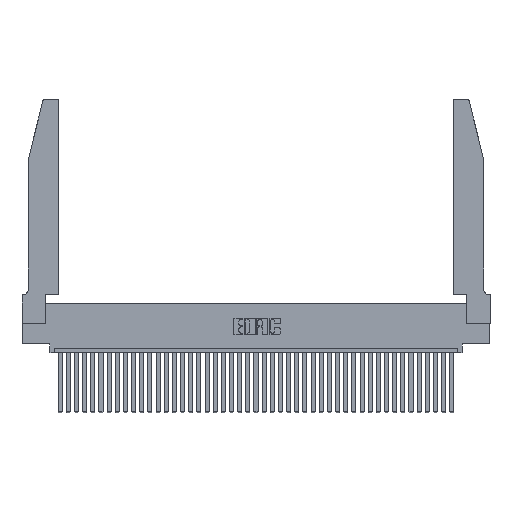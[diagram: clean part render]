
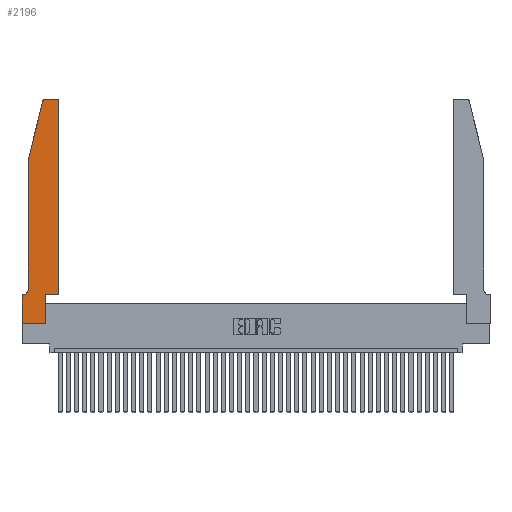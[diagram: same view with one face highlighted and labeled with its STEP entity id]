
A CAD part, top view. The second image highlights one B-rep face of the part: STEP entity #2196.
In plain terms, the highlighted planar face has unit normal (0, 0, 1).
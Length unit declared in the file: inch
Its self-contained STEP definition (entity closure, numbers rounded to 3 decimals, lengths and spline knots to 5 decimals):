
#500 = LINE ( 'NONE', #21204, #25167 ) ;
#563 = VERTEX_POINT ( 'NONE', #28806 ) ;
#975 = VECTOR ( 'NONE', #16520, 39.37008 ) ;
#1058 = EDGE_CURVE ( 'NONE', #33001, #15711, #18841, .T. ) ;
#1195 = ORIENTED_EDGE ( 'NONE', *, *, #20455, .T. ) ;
#1281 = EDGE_CURVE ( 'NONE', #563, #17294, #22710, .T. ) ;
#1528 = LINE ( 'NONE', #12996, #8435 ) ;
#2046 = ORIENTED_EDGE ( 'NONE', *, *, #39128, .T. ) ;
#2063 = CARTESIAN_POINT ( 'NONE',  ( 0.0755, 2., 0.37 ) ) ;
#2196 = ADVANCED_FACE ( 'NONE', ( #28555 ), #40489, .T. ) ;
#2417 = DIRECTION ( 'NONE',  ( 0., -1., 0. ) ) ;
#2602 = DIRECTION ( 'NONE',  ( 1., 0., 0. ) ) ;
#2818 = EDGE_CURVE ( 'NONE', #26857, #16723, #28489, .T. ) ;
#2832 = VERTEX_POINT ( 'NONE', #28249 ) ;
#2904 = ORIENTED_EDGE ( 'NONE', *, *, #22901, .T. ) ;
#3601 = CARTESIAN_POINT ( 'NONE',  ( 0.4505, 2.72, 0.37 ) ) ;
#4555 = EDGE_LOOP ( 'NONE', ( #2046, #27588, #8242, #13782, #1195, #13633, #35227, #15283, #33501, #24519, #2904, #5033 ) ) ;
#5033 = ORIENTED_EDGE ( 'NONE', *, *, #39528, .T. ) ;
#5931 = CIRCLE ( 'NONE', #22751, 0.03 ) ;
#6778 = AXIS2_PLACEMENT_3D ( 'NONE', #17816, #39734, #20983 ) ;
#8242 = ORIENTED_EDGE ( 'NONE', *, *, #39229, .T. ) ;
#8435 = VECTOR ( 'NONE', #37019, 39.37008 ) ;
#8724 = LINE ( 'NONE', #11766, #22927 ) ;
#9112 = EDGE_CURVE ( 'NONE', #15711, #29681, #8724, .T. ) ;
#11602 = DIRECTION ( 'NONE',  ( 1., 0., 0. ) ) ;
#11725 = VERTEX_POINT ( 'NONE', #21188 ) ;
#11766 = CARTESIAN_POINT ( 'NONE',  ( 0., 0., 0.37 ) ) ;
#11880 = VECTOR ( 'NONE', #16425, 39.37008 ) ;
#11906 = DIRECTION ( 'NONE',  ( 0., 0., 1. ) ) ;
#12026 = DIRECTION ( 'NONE',  ( 0., -1., 0. ) ) ;
#12458 = CARTESIAN_POINT ( 'NONE',  ( 0., 0., 0.37 ) ) ;
#12576 = DIRECTION ( 'NONE',  ( 1., 0., 0. ) ) ;
#12996 = CARTESIAN_POINT ( 'NONE',  ( 0.2605, 2.75, 0.37 ) ) ;
#13296 = DIRECTION ( 'NONE',  ( 0., 1., 0. ) ) ;
#13633 = ORIENTED_EDGE ( 'NONE', *, *, #1058, .T. ) ;
#13782 = ORIENTED_EDGE ( 'NONE', *, *, #38468, .T. ) ;
#15283 = ORIENTED_EDGE ( 'NONE', *, *, #18341, .T. ) ;
#15711 = VERTEX_POINT ( 'NONE', #21183 ) ;
#16425 = DIRECTION ( 'NONE',  ( -0.239, -0.971, 0. ) ) ;
#16520 = DIRECTION ( 'NONE',  ( 0., 1., 0. ) ) ;
#16723 = VERTEX_POINT ( 'NONE', #35335 ) ;
#16846 = CARTESIAN_POINT ( 'NONE',  ( 0.4205, 2.75, 0.37 ) ) ;
#16975 = CARTESIAN_POINT ( 'NONE',  ( 0., 0., 0.37 ) ) ;
#17267 = VECTOR ( 'NONE', #13296, 39.37008 ) ;
#17294 = VERTEX_POINT ( 'NONE', #38353 ) ;
#17816 = CARTESIAN_POINT ( 'NONE',  ( 0.0055, 0.42, 0.37 ) ) ;
#18111 = AXIS2_PLACEMENT_3D ( 'NONE', #37094, #11906, #18337 ) ;
#18337 = DIRECTION ( 'NONE',  ( 1., 0., 0. ) ) ;
#18341 = EDGE_CURVE ( 'NONE', #29681, #26857, #22492, .T. ) ;
#18841 = LINE ( 'NONE', #33192, #26197 ) ;
#19548 = VECTOR ( 'NONE', #12576, 39.37008 ) ;
#20455 = EDGE_CURVE ( 'NONE', #2832, #33001, #34054, .T. ) ;
#20983 = DIRECTION ( 'NONE',  ( -1., 0., 0. ) ) ;
#21183 = CARTESIAN_POINT ( 'NONE',  ( 0., 0.35, 0.37 ) ) ;
#21188 = CARTESIAN_POINT ( 'NONE',  ( 0.4505, 0.35, 0.37 ) ) ;
#21204 = CARTESIAN_POINT ( 'NONE',  ( 0.0755, 2., 0.37 ) ) ;
#22492 = LINE ( 'NONE', #12458, #19548 ) ;
#22710 = CIRCLE ( 'NONE', #18111, 0.03 ) ;
#22751 = AXIS2_PLACEMENT_3D ( 'NONE', #33387, #40160, #2602 ) ;
#22901 = EDGE_CURVE ( 'NONE', #11725, #30579, #29033, .T. ) ;
#22927 = VECTOR ( 'NONE', #2417, 39.37008 ) ;
#24519 = ORIENTED_EDGE ( 'NONE', *, *, #25457, .T. ) ;
#24698 = CARTESIAN_POINT ( 'NONE',  ( 0.2865, 0., 0.37 ) ) ;
#24915 = DIRECTION ( 'NONE',  ( 1., 0., 0. ) ) ;
#25123 = CARTESIAN_POINT ( 'NONE',  ( 0.4505, 0.35, 0.37 ) ) ;
#25167 = VECTOR ( 'NONE', #12026, 39.37008 ) ;
#25457 = EDGE_CURVE ( 'NONE', #16723, #11725, #30894, .T. ) ;
#26197 = VECTOR ( 'NONE', #30367, 39.37008 ) ;
#26857 = VERTEX_POINT ( 'NONE', #24698 ) ;
#27588 = ORIENTED_EDGE ( 'NONE', *, *, #1281, .T. ) ;
#27616 = CARTESIAN_POINT ( 'NONE',  ( 0.0055, 0.35, 0.37 ) ) ;
#27873 = AXIS2_PLACEMENT_3D ( 'NONE', #37576, #34389, #24915 ) ;
#28249 = CARTESIAN_POINT ( 'NONE',  ( 0.0755, 0.42, 0.37 ) ) ;
#28489 = LINE ( 'NONE', #34662, #975 ) ;
#28555 = FACE_OUTER_BOUND ( 'NONE', #4555, .T. ) ;
#28806 = CARTESIAN_POINT ( 'NONE',  ( 0.284, 2.75, 0.37 ) ) ;
#29033 = LINE ( 'NONE', #25123, #17267 ) ;
#29681 = VERTEX_POINT ( 'NONE', #16975 ) ;
#29723 = VERTEX_POINT ( 'NONE', #2063 ) ;
#30367 = DIRECTION ( 'NONE',  ( -1., 0., 0. ) ) ;
#30579 = VERTEX_POINT ( 'NONE', #3601 ) ;
#30894 = LINE ( 'NONE', #36380, #36254 ) ;
#32357 = LINE ( 'NONE', #35148, #11880 ) ;
#33001 = VERTEX_POINT ( 'NONE', #27616 ) ;
#33192 = CARTESIAN_POINT ( 'NONE',  ( 0.0755, 0.35, 0.37 ) ) ;
#33387 = CARTESIAN_POINT ( 'NONE',  ( 0.4205, 2.72, 0.37 ) ) ;
#33501 = ORIENTED_EDGE ( 'NONE', *, *, #2818, .T. ) ;
#34054 = CIRCLE ( 'NONE', #6778, 0.07 ) ;
#34389 = DIRECTION ( 'NONE',  ( 0., 0., 1. ) ) ;
#34662 = CARTESIAN_POINT ( 'NONE',  ( 0.2865, 0.35, 0.37 ) ) ;
#35148 = CARTESIAN_POINT ( 'NONE',  ( 0.0755, 2., 0.37 ) ) ;
#35227 = ORIENTED_EDGE ( 'NONE', *, *, #9112, .T. ) ;
#35335 = CARTESIAN_POINT ( 'NONE',  ( 0.2865, 0.35, 0.37 ) ) ;
#36254 = VECTOR ( 'NONE', #11602, 39.37008 ) ;
#36380 = CARTESIAN_POINT ( 'NONE',  ( 0.4505, 0.35, 0.37 ) ) ;
#37019 = DIRECTION ( 'NONE',  ( -1., 0., 0. ) ) ;
#37094 = CARTESIAN_POINT ( 'NONE',  ( 0.284, 2.72, 0.37 ) ) ;
#37576 = CARTESIAN_POINT ( 'NONE',  ( 0., 0.35, 0.37 ) ) ;
#38353 = CARTESIAN_POINT ( 'NONE',  ( 0.25487, 2.72718, 0.37 ) ) ;
#38468 = EDGE_CURVE ( 'NONE', #29723, #2832, #500, .T. ) ;
#39128 = EDGE_CURVE ( 'NONE', #40040, #563, #1528, .T. ) ;
#39229 = EDGE_CURVE ( 'NONE', #17294, #29723, #32357, .T. ) ;
#39528 = EDGE_CURVE ( 'NONE', #30579, #40040, #5931, .T. ) ;
#39734 = DIRECTION ( 'NONE',  ( 0., 0., -1. ) ) ;
#40040 = VERTEX_POINT ( 'NONE', #16846 ) ;
#40160 = DIRECTION ( 'NONE',  ( 0., 0., 1. ) ) ;
#40489 = PLANE ( 'NONE',  #27873 ) ;
